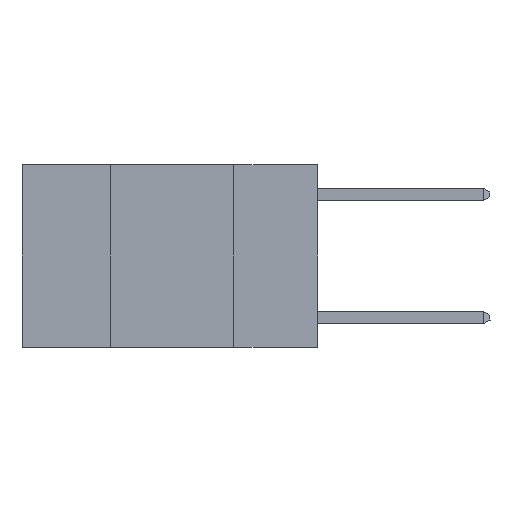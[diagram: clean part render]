
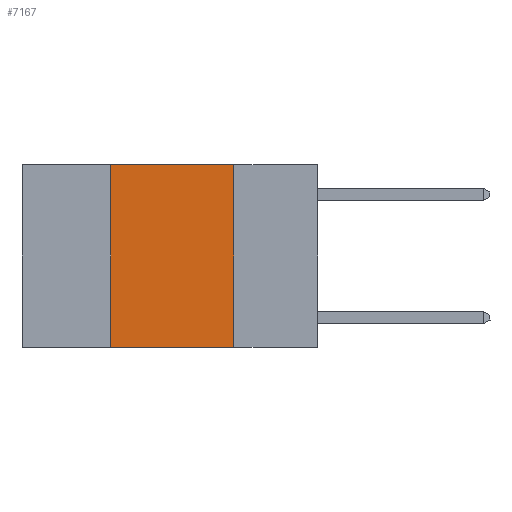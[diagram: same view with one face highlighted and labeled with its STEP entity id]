
A CAD part, left-side view. The second image highlights one B-rep face of the part: STEP entity #7167.
In plain terms, the highlighted planar face has unit normal (-1, 0, 0).
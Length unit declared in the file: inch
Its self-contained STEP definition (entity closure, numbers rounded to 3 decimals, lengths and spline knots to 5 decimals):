
#178 = EDGE_LOOP ( 'NONE', ( #503, #5910, #6240, #8897 ) ) ;
#503 = ORIENTED_EDGE ( 'NONE', *, *, #4617, .F. ) ;
#743 = CARTESIAN_POINT ( 'NONE',  ( 0., 0.6, -0.37 ) ) ;
#1366 = DIRECTION ( 'NONE',  ( 0., 0., -1. ) ) ;
#2055 = VECTOR ( 'NONE', #7088, 39.37008 ) ;
#2098 = VECTOR ( 'NONE', #9898, 39.37008 ) ;
#2950 = CARTESIAN_POINT ( 'NONE',  ( 0., 0.17, 0. ) ) ;
#3666 = CARTESIAN_POINT ( 'NONE',  ( 0., 0.17, -0.37 ) ) ;
#3921 = EDGE_CURVE ( 'NONE', #12074, #6036, #12491, .T. ) ;
#4386 = PLANE ( 'NONE',  #8706 ) ;
#4617 = EDGE_CURVE ( 'NONE', #12011, #6036, #12609, .T. ) ;
#5067 = CARTESIAN_POINT ( 'NONE',  ( 0., 0.42, -0.37 ) ) ;
#5396 = CARTESIAN_POINT ( 'NONE',  ( 0., 0.6, 0. ) ) ;
#5910 = ORIENTED_EDGE ( 'NONE', *, *, #12053, .F. ) ;
#6036 = VERTEX_POINT ( 'NONE', #3666 ) ;
#6068 = CARTESIAN_POINT ( 'NONE',  ( 0., 0.6, 0. ) ) ;
#6240 = ORIENTED_EDGE ( 'NONE', *, *, #11029, .F. ) ;
#7088 = DIRECTION ( 'NONE',  ( 0., -1., 0. ) ) ;
#7167 = ADVANCED_FACE ( 'NONE', ( #11985 ), #4386, .F. ) ;
#7413 = LINE ( 'NONE', #6068, #2055 ) ;
#7414 = DIRECTION ( 'NONE',  ( 1., 0., 0. ) ) ;
#7792 = CARTESIAN_POINT ( 'NONE',  ( 0., 0.42, 0. ) ) ;
#8706 = AXIS2_PLACEMENT_3D ( 'NONE', #5396, #7414, #1366 ) ;
#8801 = DIRECTION ( 'NONE',  ( 0., 0., 1. ) ) ;
#8863 = CARTESIAN_POINT ( 'NONE',  ( 0., 0.17, 0. ) ) ;
#8897 = ORIENTED_EDGE ( 'NONE', *, *, #3921, .T. ) ;
#9003 = VECTOR ( 'NONE', #8801, 39.37008 ) ;
#9334 = LINE ( 'NONE', #7792, #9003 ) ;
#9825 = DIRECTION ( 'NONE',  ( 0., -1., 0. ) ) ;
#9898 = DIRECTION ( 'NONE',  ( 0., 0., -1. ) ) ;
#10270 = VECTOR ( 'NONE', #9825, 39.37008 ) ;
#10500 = VERTEX_POINT ( 'NONE', #11900 ) ;
#11029 = EDGE_CURVE ( 'NONE', #12074, #10500, #9334, .T. ) ;
#11900 = CARTESIAN_POINT ( 'NONE',  ( 0., 0.42, 0. ) ) ;
#11985 = FACE_OUTER_BOUND ( 'NONE', #178, .T. ) ;
#12011 = VERTEX_POINT ( 'NONE', #2950 ) ;
#12053 = EDGE_CURVE ( 'NONE', #10500, #12011, #7413, .T. ) ;
#12074 = VERTEX_POINT ( 'NONE', #5067 ) ;
#12491 = LINE ( 'NONE', #743, #10270 ) ;
#12609 = LINE ( 'NONE', #8863, #2098 ) ;
